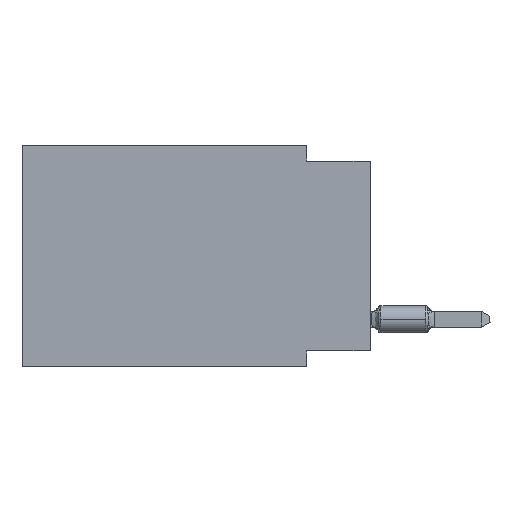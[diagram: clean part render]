
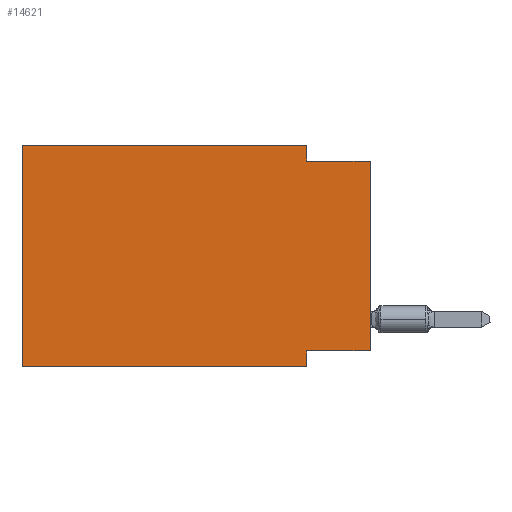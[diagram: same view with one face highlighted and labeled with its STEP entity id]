
A CAD part, left-side view. The second image highlights one B-rep face of the part: STEP entity #14621.
In plain terms, the highlighted planar face has unit normal (-1, 0, 0).
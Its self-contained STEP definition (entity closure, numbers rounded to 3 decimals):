
#302 = FACE_OUTER_BOUND ( 'NONE', #17863, .T. ) ;
#3021 = DIRECTION ( 'NONE',  ( 0., 0., -1. ) ) ;
#4178 = EDGE_CURVE ( 'NONE', #50815, #31132, #64179, .T. ) ;
#5324 = VECTOR ( 'NONE', #57272, 1000. ) ;
#7054 = CARTESIAN_POINT ( 'NONE',  ( 0., 0., -8.255 ) ) ;
#7873 = CARTESIAN_POINT ( 'NONE',  ( 0., 2.54, -8.89 ) ) ;
#9157 = EDGE_CURVE ( 'NONE', #50815, #10783, #25128, .T. ) ;
#10026 = EDGE_CURVE ( 'NONE', #10783, #69122, #25220, .T. ) ;
#10783 = VERTEX_POINT ( 'NONE', #22470 ) ;
#11202 = VECTOR ( 'NONE', #58945, 1000. ) ;
#12640 = VERTEX_POINT ( 'NONE', #63386 ) ;
#13992 = ORIENTED_EDGE ( 'NONE', *, *, #4178, .T. ) ;
#14621 = ADVANCED_FACE ( 'NONE', ( #302 ), #58673, .F. ) ;
#14624 = CARTESIAN_POINT ( 'NONE',  ( 0., 2.54, -8.89 ) ) ;
#15143 = VECTOR ( 'NONE', #3021, 1000. ) ;
#15238 = DIRECTION ( 'NONE',  ( 0., 0., 1. ) ) ;
#17863 = EDGE_LOOP ( 'NONE', ( #59936, #52359, #38498, #40876, #61106, #13992, #28501, #39376 ) ) ;
#18800 = EDGE_CURVE ( 'NONE', #12640, #31132, #62493, .T. ) ;
#19430 = LINE ( 'NONE', #28913, #15143 ) ;
#19594 = VECTOR ( 'NONE', #15238, 1000. ) ;
#22176 = VERTEX_POINT ( 'NONE', #49377 ) ;
#22470 = CARTESIAN_POINT ( 'NONE',  ( 0., 13.97, 0. ) ) ;
#25128 = LINE ( 'NONE', #56935, #25708 ) ;
#25220 = LINE ( 'NONE', #46902, #57043 ) ;
#25708 = VECTOR ( 'NONE', #35620, 1000. ) ;
#26104 = DIRECTION ( 'NONE',  ( 0., -1., 0. ) ) ;
#28501 = ORIENTED_EDGE ( 'NONE', *, *, #18800, .F. ) ;
#28913 = CARTESIAN_POINT ( 'NONE',  ( 0., 2.54, 0. ) ) ;
#31132 = VERTEX_POINT ( 'NONE', #7873 ) ;
#31549 = CARTESIAN_POINT ( 'NONE',  ( 0., 2.54, -0.635 ) ) ;
#35170 = CARTESIAN_POINT ( 'NONE',  ( 0., 2.54, 0. ) ) ;
#35620 = DIRECTION ( 'NONE',  ( 0., 0., 1. ) ) ;
#36696 = DIRECTION ( 'NONE',  ( 0., 1., 0. ) ) ;
#37019 = DIRECTION ( 'NONE',  ( 1., 0., 0. ) ) ;
#37291 = CARTESIAN_POINT ( 'NONE',  ( 0., 13.97, -8.89 ) ) ;
#37639 = LINE ( 'NONE', #63845, #11202 ) ;
#38322 = VECTOR ( 'NONE', #26104, 1000. ) ;
#38498 = ORIENTED_EDGE ( 'NONE', *, *, #43786, .F. ) ;
#39376 = ORIENTED_EDGE ( 'NONE', *, *, #62738, .F. ) ;
#40876 = ORIENTED_EDGE ( 'NONE', *, *, #10026, .F. ) ;
#41950 = CARTESIAN_POINT ( 'NONE',  ( 0., 0., -8.255 ) ) ;
#42260 = CARTESIAN_POINT ( 'NONE',  ( 0., 13.97, 0. ) ) ;
#43786 = EDGE_CURVE ( 'NONE', #69122, #62272, #19430, .T. ) ;
#46902 = CARTESIAN_POINT ( 'NONE',  ( 0., 13.97, 0. ) ) ;
#47844 = VECTOR ( 'NONE', #36696, 1000. ) ;
#49377 = CARTESIAN_POINT ( 'NONE',  ( 0., 0., -0.635 ) ) ;
#50815 = VERTEX_POINT ( 'NONE', #61439 ) ;
#51509 = EDGE_CURVE ( 'NONE', #54466, #22176, #52984, .T. ) ;
#52359 = ORIENTED_EDGE ( 'NONE', *, *, #65088, .F. ) ;
#52984 = LINE ( 'NONE', #63107, #19594 ) ;
#54466 = VERTEX_POINT ( 'NONE', #7054 ) ;
#56935 = CARTESIAN_POINT ( 'NONE',  ( 0., 13.97, 0. ) ) ;
#57043 = VECTOR ( 'NONE', #68206, 1000. ) ;
#57272 = DIRECTION ( 'NONE',  ( 0., 0., -1. ) ) ;
#57980 = DIRECTION ( 'NONE',  ( 0., 0., -1. ) ) ;
#58673 = PLANE ( 'NONE',  #61389 ) ;
#58945 = DIRECTION ( 'NONE',  ( 0., -1., 0. ) ) ;
#59936 = ORIENTED_EDGE ( 'NONE', *, *, #51509, .T. ) ;
#61106 = ORIENTED_EDGE ( 'NONE', *, *, #9157, .F. ) ;
#61389 = AXIS2_PLACEMENT_3D ( 'NONE', #42260, #37019, #57980 ) ;
#61439 = CARTESIAN_POINT ( 'NONE',  ( 0., 13.97, -8.89 ) ) ;
#62272 = VERTEX_POINT ( 'NONE', #31549 ) ;
#62493 = LINE ( 'NONE', #14624, #5324 ) ;
#62738 = EDGE_CURVE ( 'NONE', #54466, #12640, #68499, .T. ) ;
#63107 = CARTESIAN_POINT ( 'NONE',  ( 0., 0., 0. ) ) ;
#63386 = CARTESIAN_POINT ( 'NONE',  ( 0., 2.54, -8.255 ) ) ;
#63845 = CARTESIAN_POINT ( 'NONE',  ( 0., 0., -0.635 ) ) ;
#64179 = LINE ( 'NONE', #37291, #38322 ) ;
#65088 = EDGE_CURVE ( 'NONE', #62272, #22176, #37639, .T. ) ;
#68206 = DIRECTION ( 'NONE',  ( 0., -1., 0. ) ) ;
#68499 = LINE ( 'NONE', #41950, #47844 ) ;
#69122 = VERTEX_POINT ( 'NONE', #35170 ) ;
